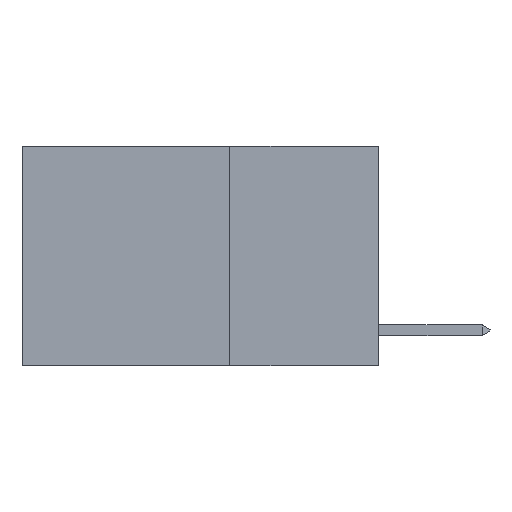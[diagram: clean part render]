
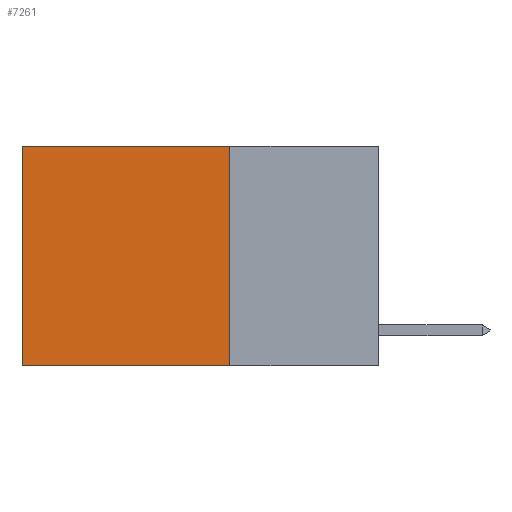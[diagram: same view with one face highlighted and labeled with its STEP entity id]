
A CAD part, left-side view. The second image highlights one B-rep face of the part: STEP entity #7261.
In plain terms, the highlighted planar face has unit normal (-1, 0, 0).
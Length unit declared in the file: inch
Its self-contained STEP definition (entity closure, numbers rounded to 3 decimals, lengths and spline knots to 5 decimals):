
#280 = VERTEX_POINT ( 'NONE', #12512 ) ;
#396 = LINE ( 'NONE', #12975, #3066 ) ;
#415 = ORIENTED_EDGE ( 'NONE', *, *, #8519, .F. ) ;
#611 = ORIENTED_EDGE ( 'NONE', *, *, #6566, .F. ) ;
#1501 = VECTOR ( 'NONE', #3834, 39.37008 ) ;
#1600 = CARTESIAN_POINT ( 'NONE',  ( 0.2625, 0.25, 0. ) ) ;
#1774 = ORIENTED_EDGE ( 'NONE', *, *, #14431, .T. ) ;
#2770 = DIRECTION ( 'NONE',  ( 0., 1., 0. ) ) ;
#3066 = VECTOR ( 'NONE', #4067, 39.37008 ) ;
#3101 = CARTESIAN_POINT ( 'NONE',  ( 0.2625, 0.6, 0. ) ) ;
#3154 = LINE ( 'NONE', #6128, #8807 ) ;
#3834 = DIRECTION ( 'NONE',  ( 0., 0., -1. ) ) ;
#3965 = PLANE ( 'NONE',  #5956 ) ;
#4067 = DIRECTION ( 'NONE',  ( 0., 0., -1. ) ) ;
#4365 = VERTEX_POINT ( 'NONE', #3101 ) ;
#4910 = VERTEX_POINT ( 'NONE', #12113 ) ;
#5008 = DIRECTION ( 'NONE',  ( 0., 1., 0. ) ) ;
#5084 = DIRECTION ( 'NONE',  ( 1., 0., 0. ) ) ;
#5504 = ORIENTED_EDGE ( 'NONE', *, *, #9530, .T. ) ;
#5627 = VECTOR ( 'NONE', #2770, 39.37008 ) ;
#5956 = AXIS2_PLACEMENT_3D ( 'NONE', #11803, #5084, #12926 ) ;
#6128 = CARTESIAN_POINT ( 'NONE',  ( 0.2625, 0.25, -0.37 ) ) ;
#6566 = EDGE_CURVE ( 'NONE', #11696, #4910, #3154, .T. ) ;
#7261 = ADVANCED_FACE ( 'NONE', ( #13483 ), #3965, .F. ) ;
#7276 = CARTESIAN_POINT ( 'NONE',  ( 0.2625, 0.25, 0. ) ) ;
#7776 = CARTESIAN_POINT ( 'NONE',  ( 0.2625, 0.25, -0.37 ) ) ;
#8519 = EDGE_CURVE ( 'NONE', #280, #11696, #10470, .T. ) ;
#8637 = LINE ( 'NONE', #7276, #5627 ) ;
#8807 = VECTOR ( 'NONE', #5008, 39.37008 ) ;
#9077 = EDGE_LOOP ( 'NONE', ( #5504, #611, #415, #1774 ) ) ;
#9530 = EDGE_CURVE ( 'NONE', #4365, #4910, #396, .T. ) ;
#10470 = LINE ( 'NONE', #1600, #1501 ) ;
#11696 = VERTEX_POINT ( 'NONE', #7776 ) ;
#11803 = CARTESIAN_POINT ( 'NONE',  ( 0.2625, 0.25, 0. ) ) ;
#12113 = CARTESIAN_POINT ( 'NONE',  ( 0.2625, 0.6, -0.37 ) ) ;
#12512 = CARTESIAN_POINT ( 'NONE',  ( 0.2625, 0.25, 0. ) ) ;
#12926 = DIRECTION ( 'NONE',  ( 0., 0., -1. ) ) ;
#12975 = CARTESIAN_POINT ( 'NONE',  ( 0.2625, 0.6, 0. ) ) ;
#13483 = FACE_OUTER_BOUND ( 'NONE', #9077, .T. ) ;
#14431 = EDGE_CURVE ( 'NONE', #280, #4365, #8637, .T. ) ;
